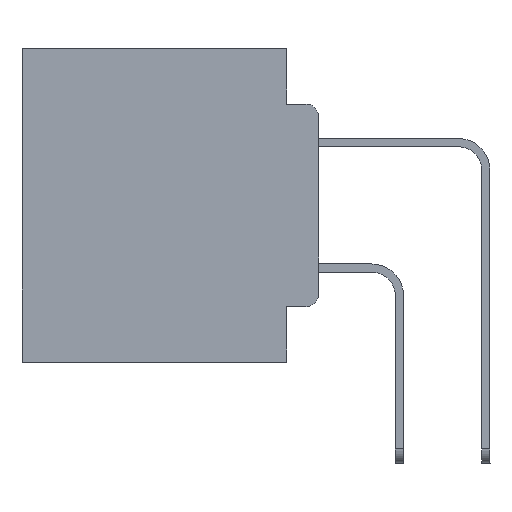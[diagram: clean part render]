
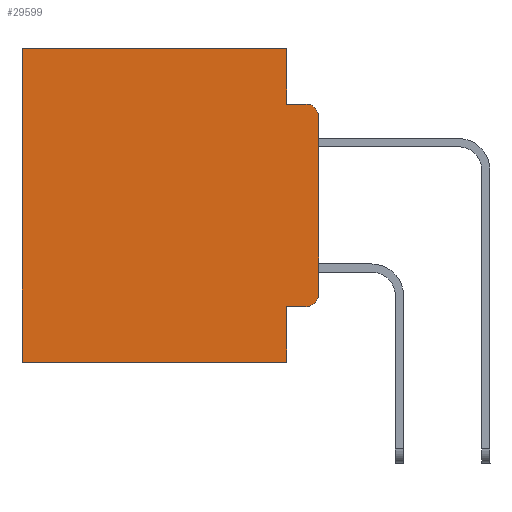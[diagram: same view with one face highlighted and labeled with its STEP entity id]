
A CAD part, left-side view. The second image highlights one B-rep face of the part: STEP entity #29599.
In plain terms, the highlighted planar face has unit normal (-1, 0, 0).
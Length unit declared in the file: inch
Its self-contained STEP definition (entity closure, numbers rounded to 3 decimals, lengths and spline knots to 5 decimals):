
#1382 = ORIENTED_EDGE ( 'NONE', *, *, #1460, .F. ) ;
#1460 = EDGE_CURVE ( 'NONE', #26762, #3392, #10763, .T. ) ;
#1606 = VECTOR ( 'NONE', #4301, 39.37008 ) ;
#1982 = CARTESIAN_POINT ( 'NONE',  ( 0.298, 0., -0.5 ) ) ;
#2008 = DIRECTION ( 'NONE',  ( 0., 0., -1. ) ) ;
#2344 = CARTESIAN_POINT ( 'NONE',  ( 0.298, 0.051, -0.4115 ) ) ;
#2754 = EDGE_CURVE ( 'NONE', #20561, #18071, #18614, .T. ) ;
#3073 = EDGE_CURVE ( 'NONE', #3392, #6004, #28646, .T. ) ;
#3392 = VERTEX_POINT ( 'NONE', #14137 ) ;
#3493 = DIRECTION ( 'NONE',  ( 0., -1., 0. ) ) ;
#4301 = DIRECTION ( 'NONE',  ( 0., 1., 0. ) ) ;
#4555 = DIRECTION ( 'NONE',  ( 0., 1., 0. ) ) ;
#4590 = VECTOR ( 'NONE', #9399, 39.37008 ) ;
#5878 = ORIENTED_EDGE ( 'NONE', *, *, #7252, .F. ) ;
#6004 = VERTEX_POINT ( 'NONE', #10910 ) ;
#6861 = LINE ( 'NONE', #17984, #18428 ) ;
#7118 = CARTESIAN_POINT ( 'NONE',  ( 0.298, 0.473, 0. ) ) ;
#7252 = EDGE_CURVE ( 'NONE', #12107, #9256, #21809, .T. ) ;
#7570 = EDGE_CURVE ( 'NONE', #26762, #7895, #25369, .T. ) ;
#7601 = DIRECTION ( 'NONE',  ( 0., 0., -1. ) ) ;
#7895 = VERTEX_POINT ( 'NONE', #7118 ) ;
#8144 = CARTESIAN_POINT ( 'NONE',  ( 0.298, 0., -0.3915 ) ) ;
#8637 = DIRECTION ( 'NONE',  ( 0., 0., -1. ) ) ;
#8926 = DIRECTION ( 'NONE',  ( -1., 0., 0. ) ) ;
#9256 = VERTEX_POINT ( 'NONE', #8144 ) ;
#9399 = DIRECTION ( 'NONE',  ( 0., 0., -1. ) ) ;
#9593 = CARTESIAN_POINT ( 'NONE',  ( 0.298, 0.02, -0.1085 ) ) ;
#9736 = DIRECTION ( 'NONE',  ( 0., 0., -1. ) ) ;
#10015 = EDGE_CURVE ( 'NONE', #18589, #9256, #22414, .T. ) ;
#10130 = CARTESIAN_POINT ( 'NONE',  ( 0.298, 0.051, 0. ) ) ;
#10629 = CARTESIAN_POINT ( 'NONE',  ( 0.298, 0.02, -0.4115 ) ) ;
#10763 = LINE ( 'NONE', #10130, #16874 ) ;
#10866 = LINE ( 'NONE', #16249, #4590 ) ;
#10910 = CARTESIAN_POINT ( 'NONE',  ( 0.298, 0.02, -0.0885 ) ) ;
#11125 = CARTESIAN_POINT ( 'NONE',  ( 0.298, 0., 0. ) ) ;
#11445 = VECTOR ( 'NONE', #3493, 39.37008 ) ;
#11925 = DIRECTION ( 'NONE',  ( 0., 0., -1. ) ) ;
#12107 = VERTEX_POINT ( 'NONE', #18693 ) ;
#12210 = EDGE_LOOP ( 'NONE', ( #5878, #24785, #23100, #1382, #16469, #23735, #15051, #28256, #22338, #18541 ) ) ;
#12546 = CIRCLE ( 'NONE', #25843, 0.02 ) ;
#13107 = EDGE_CURVE ( 'NONE', #13940, #18589, #6861, .T. ) ;
#13495 = DIRECTION ( 'NONE',  ( 0., -1., 0. ) ) ;
#13704 = CARTESIAN_POINT ( 'NONE',  ( 0.298, 0.051, 0. ) ) ;
#13741 = PLANE ( 'NONE',  #27943 ) ;
#13940 = VERTEX_POINT ( 'NONE', #2344 ) ;
#14137 = CARTESIAN_POINT ( 'NONE',  ( 0.298, 0.051, -0.0885 ) ) ;
#14184 = VECTOR ( 'NONE', #7601, 39.37008 ) ;
#14634 = CARTESIAN_POINT ( 'NONE',  ( 0.298, 0.473, 0. ) ) ;
#15051 = ORIENTED_EDGE ( 'NONE', *, *, #2754, .F. ) ;
#15620 = EDGE_CURVE ( 'NONE', #12107, #6004, #12546, .T. ) ;
#15769 = CARTESIAN_POINT ( 'NONE',  ( 0.298, 0.051, -0.5 ) ) ;
#16035 = DIRECTION ( 'NONE',  ( 1., 0., 0. ) ) ;
#16249 = CARTESIAN_POINT ( 'NONE',  ( 0.298, 0.051, 0. ) ) ;
#16469 = ORIENTED_EDGE ( 'NONE', *, *, #7570, .T. ) ;
#16874 = VECTOR ( 'NONE', #8637, 39.37008 ) ;
#17344 = AXIS2_PLACEMENT_3D ( 'NONE', #22548, #8926, #24772 ) ;
#17895 = VECTOR ( 'NONE', #4555, 39.37008 ) ;
#17984 = CARTESIAN_POINT ( 'NONE',  ( 0.298, 0.051, -0.4115 ) ) ;
#18071 = VERTEX_POINT ( 'NONE', #24362 ) ;
#18428 = VECTOR ( 'NONE', #13495, 39.37008 ) ;
#18541 = ORIENTED_EDGE ( 'NONE', *, *, #10015, .T. ) ;
#18589 = VERTEX_POINT ( 'NONE', #10629 ) ;
#18614 = LINE ( 'NONE', #1982, #17895 ) ;
#18693 = CARTESIAN_POINT ( 'NONE',  ( 0.298, 0., -0.1085 ) ) ;
#20233 = CARTESIAN_POINT ( 'NONE',  ( 0.298, 0.051, -0.0885 ) ) ;
#20561 = VERTEX_POINT ( 'NONE', #15769 ) ;
#20699 = EDGE_CURVE ( 'NONE', #13940, #20561, #10866, .T. ) ;
#21809 = LINE ( 'NONE', #11125, #27723 ) ;
#22204 = FACE_OUTER_BOUND ( 'NONE', #12210, .T. ) ;
#22338 = ORIENTED_EDGE ( 'NONE', *, *, #13107, .T. ) ;
#22414 = CIRCLE ( 'NONE', #17344, 0.02 ) ;
#22548 = CARTESIAN_POINT ( 'NONE',  ( 0.298, 0.02, -0.3915 ) ) ;
#23100 = ORIENTED_EDGE ( 'NONE', *, *, #3073, .F. ) ;
#23735 = ORIENTED_EDGE ( 'NONE', *, *, #28139, .T. ) ;
#24362 = CARTESIAN_POINT ( 'NONE',  ( 0.298, 0.473, -0.5 ) ) ;
#24772 = DIRECTION ( 'NONE',  ( 0., 0., -1. ) ) ;
#24785 = ORIENTED_EDGE ( 'NONE', *, *, #15620, .T. ) ;
#25330 = CARTESIAN_POINT ( 'NONE',  ( 0.298, 0., 0. ) ) ;
#25369 = LINE ( 'NONE', #25330, #1606 ) ;
#25415 = DIRECTION ( 'NONE',  ( -1., 0., 0. ) ) ;
#25843 = AXIS2_PLACEMENT_3D ( 'NONE', #9593, #25415, #11925 ) ;
#26104 = LINE ( 'NONE', #14634, #14184 ) ;
#26762 = VERTEX_POINT ( 'NONE', #13704 ) ;
#27723 = VECTOR ( 'NONE', #9736, 39.37008 ) ;
#27943 = AXIS2_PLACEMENT_3D ( 'NONE', #29364, #16035, #2008 ) ;
#28139 = EDGE_CURVE ( 'NONE', #7895, #18071, #26104, .T. ) ;
#28256 = ORIENTED_EDGE ( 'NONE', *, *, #20699, .F. ) ;
#28646 = LINE ( 'NONE', #20233, #11445 ) ;
#29364 = CARTESIAN_POINT ( 'NONE',  ( 0.298, 0., 0. ) ) ;
#29599 = ADVANCED_FACE ( 'NONE', ( #22204 ), #13741, .F. ) ;
